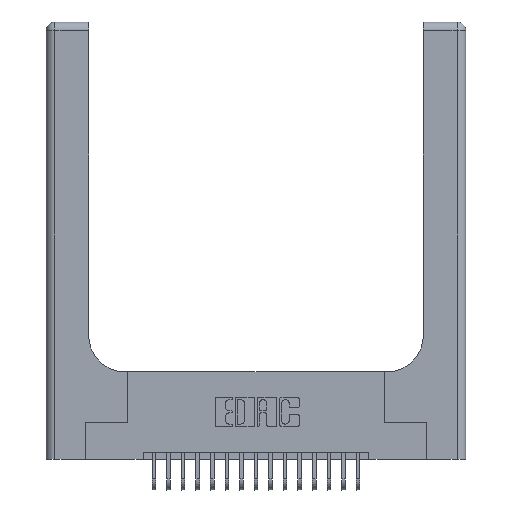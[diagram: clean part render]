
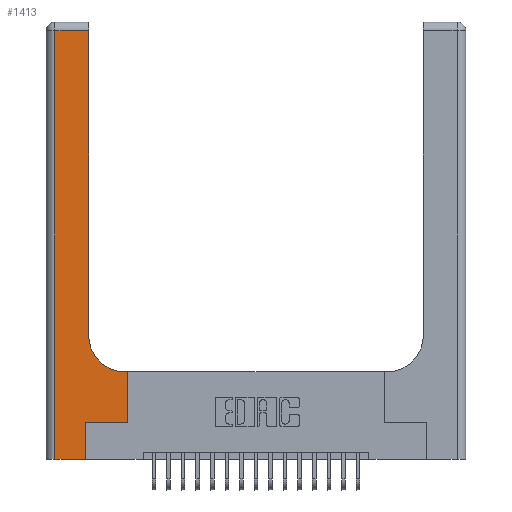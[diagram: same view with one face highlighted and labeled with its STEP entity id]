
A CAD part, top view. The second image highlights one B-rep face of the part: STEP entity #1413.
In plain terms, the highlighted planar face has unit normal (0, 0, 1).
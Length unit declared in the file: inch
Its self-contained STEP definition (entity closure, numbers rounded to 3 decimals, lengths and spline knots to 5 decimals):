
#184 = EDGE_CURVE ( 'NONE', #17867, #10274, #12282, .T. ) ;
#297 = VERTEX_POINT ( 'NONE', #18608 ) ;
#713 = VERTEX_POINT ( 'NONE', #20181 ) ;
#744 = CARTESIAN_POINT ( 'NONE',  ( 0.269, 0., 0.37 ) ) ;
#1374 = DIRECTION ( 'NONE',  ( 0., 1., 0. ) ) ;
#1413 = ADVANCED_FACE ( 'NONE', ( #12213 ), #13579, .F. ) ;
#1495 = VERTEX_POINT ( 'NONE', #10076 ) ;
#2011 = DIRECTION ( 'NONE',  ( 1., 0., 0. ) ) ;
#2097 = ORIENTED_EDGE ( 'NONE', *, *, #19537, .T. ) ;
#2486 = DIRECTION ( 'NONE',  ( 0., 1., 0. ) ) ;
#3181 = ORIENTED_EDGE ( 'NONE', *, *, #16591, .T. ) ;
#3239 = DIRECTION ( 'NONE',  ( -1., 0., 0. ) ) ;
#3389 = DIRECTION ( 'NONE',  ( 1., 0., 0. ) ) ;
#3965 = VECTOR ( 'NONE', #2011, 39.37008 ) ;
#4066 = CARTESIAN_POINT ( 'NONE',  ( 0.5585, 0.25, 0.37 ) ) ;
#4422 = CARTESIAN_POINT ( 'NONE',  ( 0.2915, 0.85, 0.37 ) ) ;
#4791 = DIRECTION ( 'NONE',  ( 0., 1., 0. ) ) ;
#4830 = DIRECTION ( 'NONE',  ( 0., 0., -1. ) ) ;
#5044 = LINE ( 'NONE', #20885, #3965 ) ;
#5139 = CARTESIAN_POINT ( 'NONE',  ( 0.5415, 0.85, 0.37 ) ) ;
#5617 = EDGE_CURVE ( 'NONE', #18950, #297, #7558, .T. ) ;
#5627 = VECTOR ( 'NONE', #1374, 39.37008 ) ;
#5795 = LINE ( 'NONE', #13808, #20840 ) ;
#5879 = VECTOR ( 'NONE', #15926, 39.37008 ) ;
#5907 = VECTOR ( 'NONE', #11365, 39.37008 ) ;
#6137 = CARTESIAN_POINT ( 'NONE',  ( 0., 2.94, 0.37 ) ) ;
#6469 = CARTESIAN_POINT ( 'NONE',  ( 0.06, 0., 0.37 ) ) ;
#6988 = EDGE_CURVE ( 'NONE', #713, #9311, #13685, .T. ) ;
#7558 = LINE ( 'NONE', #10202, #5627 ) ;
#8417 = CARTESIAN_POINT ( 'NONE',  ( 0.5585, 0.25, 0.37 ) ) ;
#8488 = DIRECTION ( 'NONE',  ( 1., 0., 0. ) ) ;
#8612 = CARTESIAN_POINT ( 'NONE',  ( 0., 3., 0.37 ) ) ;
#8964 = DIRECTION ( 'NONE',  ( 0., -1., 0. ) ) ;
#9311 = VERTEX_POINT ( 'NONE', #6469 ) ;
#10076 = CARTESIAN_POINT ( 'NONE',  ( 0.5585, 0.6, 0.37 ) ) ;
#10090 = CARTESIAN_POINT ( 'NONE',  ( 0.269, 0.25, 0.37 ) ) ;
#10202 = CARTESIAN_POINT ( 'NONE',  ( 0.2915, 3., 0.37 ) ) ;
#10274 = VERTEX_POINT ( 'NONE', #10090 ) ;
#10860 = EDGE_CURVE ( 'NONE', #14434, #18950, #11058, .T. ) ;
#10865 = LINE ( 'NONE', #8417, #17829 ) ;
#10965 = EDGE_CURVE ( 'NONE', #1495, #14434, #14010, .T. ) ;
#11058 = CIRCLE ( 'NONE', #21151, 0.25 ) ;
#11365 = DIRECTION ( 'NONE',  ( -1., 0., 0. ) ) ;
#11748 = EDGE_LOOP ( 'NONE', ( #17925, #18386, #21359, #18139, #21462, #3181, #2097, #19908, #12219 ) ) ;
#12213 = FACE_OUTER_BOUND ( 'NONE', #11748, .T. ) ;
#12219 = ORIENTED_EDGE ( 'NONE', *, *, #10860, .T. ) ;
#12282 = LINE ( 'NONE', #744, #18991 ) ;
#13409 = CARTESIAN_POINT ( 'NONE',  ( 0.06, 3., 0.37 ) ) ;
#13579 = PLANE ( 'NONE',  #15886 ) ;
#13685 = LINE ( 'NONE', #13409, #19583 ) ;
#13808 = CARTESIAN_POINT ( 'NONE',  ( 0., 0., 0.37 ) ) ;
#14010 = LINE ( 'NONE', #19136, #5879 ) ;
#14097 = CARTESIAN_POINT ( 'NONE',  ( 0.5415, 0.6, 0.37 ) ) ;
#14291 = EDGE_CURVE ( 'NONE', #9311, #17867, #5795, .T. ) ;
#14434 = VERTEX_POINT ( 'NONE', #14097 ) ;
#15886 = AXIS2_PLACEMENT_3D ( 'NONE', #8612, #4830, #3239 ) ;
#15926 = DIRECTION ( 'NONE',  ( -1., 0., 0. ) ) ;
#16089 = VERTEX_POINT ( 'NONE', #4066 ) ;
#16591 = EDGE_CURVE ( 'NONE', #10274, #16089, #5044, .T. ) ;
#17201 = DIRECTION ( 'NONE',  ( 0., 0., -1. ) ) ;
#17829 = VECTOR ( 'NONE', #4791, 39.37008 ) ;
#17867 = VERTEX_POINT ( 'NONE', #19425 ) ;
#17925 = ORIENTED_EDGE ( 'NONE', *, *, #5617, .T. ) ;
#18139 = ORIENTED_EDGE ( 'NONE', *, *, #14291, .T. ) ;
#18386 = ORIENTED_EDGE ( 'NONE', *, *, #22049, .T. ) ;
#18608 = CARTESIAN_POINT ( 'NONE',  ( 0.2915, 2.94, 0.37 ) ) ;
#18950 = VERTEX_POINT ( 'NONE', #4422 ) ;
#18991 = VECTOR ( 'NONE', #2486, 39.37008 ) ;
#19136 = CARTESIAN_POINT ( 'NONE',  ( 0.2915, 0.6, 0.37 ) ) ;
#19425 = CARTESIAN_POINT ( 'NONE',  ( 0.269, 0., 0.37 ) ) ;
#19537 = EDGE_CURVE ( 'NONE', #16089, #1495, #10865, .T. ) ;
#19583 = VECTOR ( 'NONE', #8964, 39.37008 ) ;
#19908 = ORIENTED_EDGE ( 'NONE', *, *, #10965, .T. ) ;
#20181 = CARTESIAN_POINT ( 'NONE',  ( 0.06, 2.94, 0.37 ) ) ;
#20840 = VECTOR ( 'NONE', #3389, 39.37008 ) ;
#20885 = CARTESIAN_POINT ( 'NONE',  ( 0.269, 0.25, 0.37 ) ) ;
#21151 = AXIS2_PLACEMENT_3D ( 'NONE', #5139, #17201, #8488 ) ;
#21359 = ORIENTED_EDGE ( 'NONE', *, *, #6988, .T. ) ;
#21462 = ORIENTED_EDGE ( 'NONE', *, *, #184, .T. ) ;
#21500 = LINE ( 'NONE', #6137, #5907 ) ;
#22049 = EDGE_CURVE ( 'NONE', #297, #713, #21500, .T. ) ;
